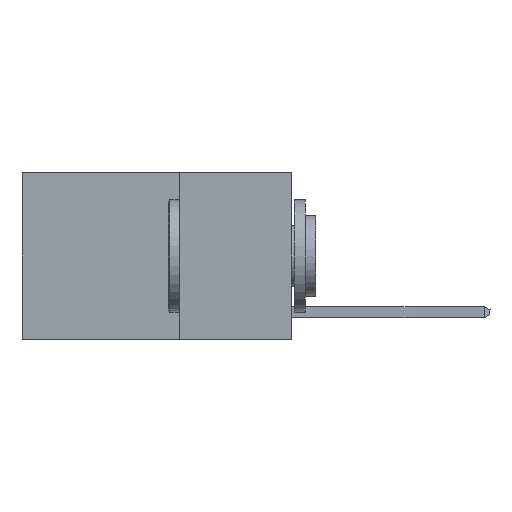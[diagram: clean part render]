
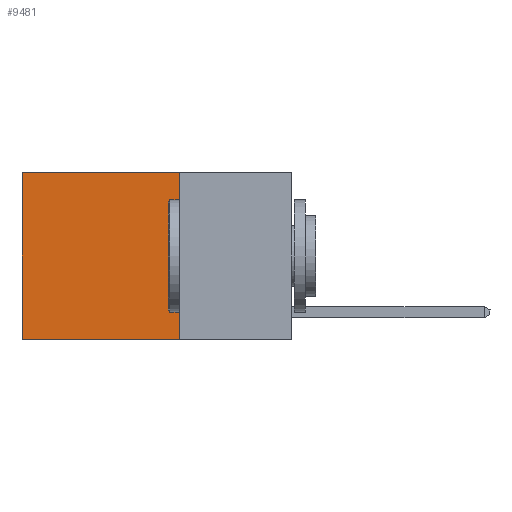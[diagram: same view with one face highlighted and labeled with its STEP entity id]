
A CAD part, left-side view. The second image highlights one B-rep face of the part: STEP entity #9481.
In plain terms, the highlighted planar face has unit normal (-1, 0, 0).
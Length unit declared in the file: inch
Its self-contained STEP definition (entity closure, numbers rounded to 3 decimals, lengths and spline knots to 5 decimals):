
#10 = AXIS2_PLACEMENT_3D ( 'NONE', #5596, #21034, #15894 ) ;
#26 = CARTESIAN_POINT ( 'NONE',  ( 0.2625, 0.6, -0.37 ) ) ;
#198 = LINE ( 'NONE', #13323, #8572 ) ;
#653 = VERTEX_POINT ( 'NONE', #26 ) ;
#753 = VERTEX_POINT ( 'NONE', #21116 ) ;
#1588 = EDGE_CURVE ( 'NONE', #8519, #653, #11961, .T. ) ;
#2946 = DIRECTION ( 'NONE',  ( 0., 0., -1. ) ) ;
#3172 = LINE ( 'NONE', #9622, #9387 ) ;
#5596 = CARTESIAN_POINT ( 'NONE',  ( 0.2625, 0.25, 0. ) ) ;
#6508 = DIRECTION ( 'NONE',  ( 0., 1., 0. ) ) ;
#7676 = DIRECTION ( 'NONE',  ( 0., 1., 0. ) ) ;
#7993 = CARTESIAN_POINT ( 'NONE',  ( 0.2625, 0.25, -0.37 ) ) ;
#8388 = CARTESIAN_POINT ( 'NONE',  ( 0.2625, 0.25, 0. ) ) ;
#8519 = VERTEX_POINT ( 'NONE', #7993 ) ;
#8572 = VECTOR ( 'NONE', #2946, 39.37008 ) ;
#8622 = CARTESIAN_POINT ( 'NONE',  ( 0.2625, 0.6, 0. ) ) ;
#8924 = PLANE ( 'NONE',  #10 ) ;
#9285 = EDGE_CURVE ( 'NONE', #753, #21748, #17007, .T. ) ;
#9387 = VECTOR ( 'NONE', #19769, 39.37008 ) ;
#9481 = ADVANCED_FACE ( 'NONE', ( #20253 ), #8924, .F. ) ;
#9622 = CARTESIAN_POINT ( 'NONE',  ( 0.2625, 0.6, 0. ) ) ;
#9811 = EDGE_CURVE ( 'NONE', #753, #8519, #198, .T. ) ;
#10160 = ORIENTED_EDGE ( 'NONE', *, *, #9285, .T. ) ;
#11153 = EDGE_LOOP ( 'NONE', ( #15704, #18131, #17338, #10160 ) ) ;
#11961 = LINE ( 'NONE', #18051, #17894 ) ;
#13323 = CARTESIAN_POINT ( 'NONE',  ( 0.2625, 0.25, 0. ) ) ;
#15704 = ORIENTED_EDGE ( 'NONE', *, *, #17206, .T. ) ;
#15894 = DIRECTION ( 'NONE',  ( 0., 0., -1. ) ) ;
#17007 = LINE ( 'NONE', #8388, #17797 ) ;
#17206 = EDGE_CURVE ( 'NONE', #21748, #653, #3172, .T. ) ;
#17338 = ORIENTED_EDGE ( 'NONE', *, *, #9811, .F. ) ;
#17797 = VECTOR ( 'NONE', #6508, 39.37008 ) ;
#17894 = VECTOR ( 'NONE', #7676, 39.37008 ) ;
#18051 = CARTESIAN_POINT ( 'NONE',  ( 0.2625, 0.25, -0.37 ) ) ;
#18131 = ORIENTED_EDGE ( 'NONE', *, *, #1588, .F. ) ;
#19769 = DIRECTION ( 'NONE',  ( 0., 0., -1. ) ) ;
#20253 = FACE_OUTER_BOUND ( 'NONE', #11153, .T. ) ;
#21034 = DIRECTION ( 'NONE',  ( 1., 0., 0. ) ) ;
#21116 = CARTESIAN_POINT ( 'NONE',  ( 0.2625, 0.25, 0. ) ) ;
#21748 = VERTEX_POINT ( 'NONE', #8622 ) ;
